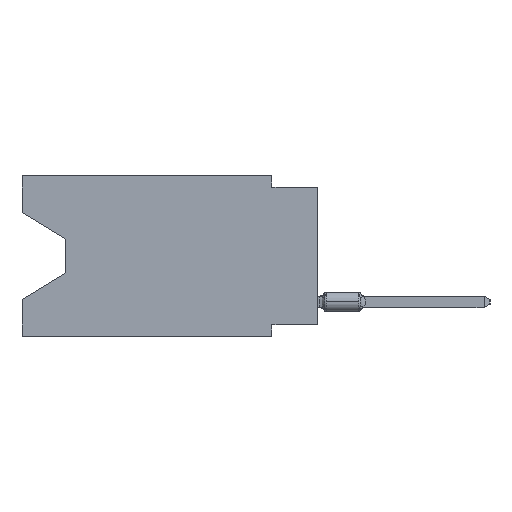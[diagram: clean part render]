
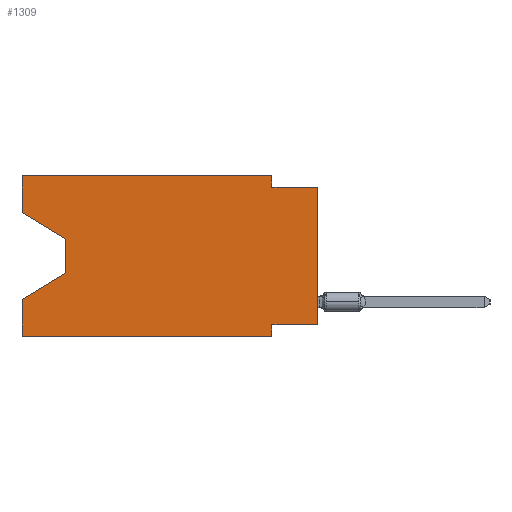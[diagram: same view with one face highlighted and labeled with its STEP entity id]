
A CAD part, left-side view. The second image highlights one B-rep face of the part: STEP entity #1309.
In plain terms, the highlighted planar face has unit normal (-1, 0, 0).
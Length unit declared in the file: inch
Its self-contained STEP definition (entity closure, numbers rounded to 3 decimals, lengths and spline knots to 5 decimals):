
#181 = ORIENTED_EDGE ( 'NONE', *, *, #13323, .T. ) ;
#307 = VECTOR ( 'NONE', #14241, 39.37008 ) ;
#564 = CARTESIAN_POINT ( 'NONE',  ( 0., 0., -0.325 ) ) ;
#871 = DIRECTION ( 'NONE',  ( 0., 0., -1. ) ) ;
#1221 = ORIENTED_EDGE ( 'NONE', *, *, #9438, .F. ) ;
#1309 = ADVANCED_FACE ( 'NONE', ( #15555 ), #1521, .F. ) ;
#1516 = EDGE_LOOP ( 'NONE', ( #21024, #16676, #6185, #19109, #11508, #5400, #8200, #181, #15451, #1221, #11687, #3195 ) ) ;
#1521 = PLANE ( 'NONE',  #21108 ) ;
#1613 = VECTOR ( 'NONE', #12825, 39.37008 ) ;
#1845 = LINE ( 'NONE', #20956, #19260 ) ;
#2079 = DIRECTION ( 'NONE',  ( 0., 0., -1. ) ) ;
#2118 = VECTOR ( 'NONE', #14619, 39.37008 ) ;
#2159 = LINE ( 'NONE', #7213, #307 ) ;
#2301 = CARTESIAN_POINT ( 'NONE',  ( 0., 0., -0.325 ) ) ;
#2612 = VERTEX_POINT ( 'NONE', #21653 ) ;
#2760 = DIRECTION ( 'NONE',  ( 0., 0., -1. ) ) ;
#2780 = VECTOR ( 'NONE', #13853, 39.37008 ) ;
#2837 = EDGE_CURVE ( 'NONE', #18678, #20106, #11973, .T. ) ;
#3013 = CARTESIAN_POINT ( 'NONE',  ( 0., 0.55, -0.212 ) ) ;
#3195 = ORIENTED_EDGE ( 'NONE', *, *, #2837, .F. ) ;
#3665 = CARTESIAN_POINT ( 'NONE',  ( 0., 0.1, -0.35 ) ) ;
#3809 = VECTOR ( 'NONE', #22788, 39.37008 ) ;
#3866 = VERTEX_POINT ( 'NONE', #10988 ) ;
#4415 = CARTESIAN_POINT ( 'NONE',  ( 0., 0.645, -0.26975 ) ) ;
#4478 = VECTOR ( 'NONE', #4640, 39.37008 ) ;
#4485 = DIRECTION ( 'NONE',  ( 0., -1., 0. ) ) ;
#4640 = DIRECTION ( 'NONE',  ( 0., 0., -1. ) ) ;
#5290 = DIRECTION ( 'NONE',  ( 0., -0.855, -0.519 ) ) ;
#5293 = EDGE_CURVE ( 'NONE', #9256, #19907, #11342, .T. ) ;
#5400 = ORIENTED_EDGE ( 'NONE', *, *, #7651, .F. ) ;
#5637 = LINE ( 'NONE', #15893, #22373 ) ;
#6131 = VECTOR ( 'NONE', #13792, 39.37008 ) ;
#6185 = ORIENTED_EDGE ( 'NONE', *, *, #18871, .T. ) ;
#6203 = VERTEX_POINT ( 'NONE', #7719 ) ;
#6368 = VERTEX_POINT ( 'NONE', #3665 ) ;
#7213 = CARTESIAN_POINT ( 'NONE',  ( 0., 0.55, -0.212 ) ) ;
#7296 = CARTESIAN_POINT ( 'NONE',  ( 0., 0.1, 0. ) ) ;
#7651 = EDGE_CURVE ( 'NONE', #10401, #6368, #5637, .T. ) ;
#7719 = CARTESIAN_POINT ( 'NONE',  ( 0., 0.1, -0.025 ) ) ;
#7851 = LINE ( 'NONE', #16500, #1613 ) ;
#7866 = EDGE_CURVE ( 'NONE', #20106, #14023, #15283, .T. ) ;
#8200 = ORIENTED_EDGE ( 'NONE', *, *, #20249, .F. ) ;
#8267 = LINE ( 'NONE', #20369, #8464 ) ;
#8464 = VECTOR ( 'NONE', #4485, 39.37008 ) ;
#8554 = CARTESIAN_POINT ( 'NONE',  ( 0., 0., 0. ) ) ;
#9256 = VERTEX_POINT ( 'NONE', #20714 ) ;
#9433 = VERTEX_POINT ( 'NONE', #564 ) ;
#9438 = EDGE_CURVE ( 'NONE', #14023, #6203, #16571, .T. ) ;
#10234 = CARTESIAN_POINT ( 'NONE',  ( 0., 0.645, 0. ) ) ;
#10401 = VERTEX_POINT ( 'NONE', #17309 ) ;
#10988 = CARTESIAN_POINT ( 'NONE',  ( 0., 0., -0.025 ) ) ;
#11066 = LINE ( 'NONE', #2301, #2118 ) ;
#11263 = EDGE_CURVE ( 'NONE', #2612, #6368, #8267, .T. ) ;
#11342 = LINE ( 'NONE', #22258, #4478 ) ;
#11508 = ORIENTED_EDGE ( 'NONE', *, *, #11263, .T. ) ;
#11687 = ORIENTED_EDGE ( 'NONE', *, *, #7866, .F. ) ;
#11973 = LINE ( 'NONE', #20702, #3809 ) ;
#12028 = LINE ( 'NONE', #8554, #2780 ) ;
#12166 = EDGE_CURVE ( 'NONE', #18678, #9256, #1845, .T. ) ;
#12452 = CARTESIAN_POINT ( 'NONE',  ( 0., 0.645, 0. ) ) ;
#12825 = DIRECTION ( 'NONE',  ( 0., -1., 0. ) ) ;
#13207 = VECTOR ( 'NONE', #13673, 39.37008 ) ;
#13323 = EDGE_CURVE ( 'NONE', #9433, #3866, #12028, .T. ) ;
#13673 = DIRECTION ( 'NONE',  ( 0., -1., 0. ) ) ;
#13792 = DIRECTION ( 'NONE',  ( 0., 0., 1. ) ) ;
#13853 = DIRECTION ( 'NONE',  ( 0., 0., 1. ) ) ;
#14023 = VERTEX_POINT ( 'NONE', #7296 ) ;
#14241 = DIRECTION ( 'NONE',  ( 0., 0.855, -0.519 ) ) ;
#14619 = DIRECTION ( 'NONE',  ( 0., 1., 0. ) ) ;
#15283 = LINE ( 'NONE', #22314, #13207 ) ;
#15451 = ORIENTED_EDGE ( 'NONE', *, *, #22483, .F. ) ;
#15555 = FACE_OUTER_BOUND ( 'NONE', #1516, .T. ) ;
#15893 = CARTESIAN_POINT ( 'NONE',  ( 0., 0.1, -0.35 ) ) ;
#16339 = CARTESIAN_POINT ( 'NONE',  ( 0., 0.1, 0. ) ) ;
#16500 = CARTESIAN_POINT ( 'NONE',  ( 0., 0., -0.025 ) ) ;
#16571 = LINE ( 'NONE', #16339, #17259 ) ;
#16676 = ORIENTED_EDGE ( 'NONE', *, *, #5293, .T. ) ;
#17259 = VECTOR ( 'NONE', #2760, 39.37008 ) ;
#17298 = CARTESIAN_POINT ( 'NONE',  ( 0., 0.645, 0. ) ) ;
#17309 = CARTESIAN_POINT ( 'NONE',  ( 0., 0.1, -0.325 ) ) ;
#17419 = EDGE_CURVE ( 'NONE', #2612, #20983, #20809, .T. ) ;
#18678 = VERTEX_POINT ( 'NONE', #20812 ) ;
#18792 = DIRECTION ( 'NONE',  ( 1., 0., 0. ) ) ;
#18871 = EDGE_CURVE ( 'NONE', #19907, #20983, #2159, .T. ) ;
#19109 = ORIENTED_EDGE ( 'NONE', *, *, #17419, .F. ) ;
#19260 = VECTOR ( 'NONE', #5290, 39.37008 ) ;
#19907 = VERTEX_POINT ( 'NONE', #3013 ) ;
#20106 = VERTEX_POINT ( 'NONE', #12452 ) ;
#20249 = EDGE_CURVE ( 'NONE', #9433, #10401, #11066, .T. ) ;
#20369 = CARTESIAN_POINT ( 'NONE',  ( 0., 0.645, -0.35 ) ) ;
#20702 = CARTESIAN_POINT ( 'NONE',  ( 0., 0.645, 0. ) ) ;
#20714 = CARTESIAN_POINT ( 'NONE',  ( 0., 0.55, -0.138 ) ) ;
#20809 = LINE ( 'NONE', #10234, #6131 ) ;
#20812 = CARTESIAN_POINT ( 'NONE',  ( 0., 0.645, -0.08025 ) ) ;
#20956 = CARTESIAN_POINT ( 'NONE',  ( 0., 0.645, -0.08025 ) ) ;
#20983 = VERTEX_POINT ( 'NONE', #4415 ) ;
#21024 = ORIENTED_EDGE ( 'NONE', *, *, #12166, .T. ) ;
#21108 = AXIS2_PLACEMENT_3D ( 'NONE', #17298, #18792, #871 ) ;
#21653 = CARTESIAN_POINT ( 'NONE',  ( 0., 0.645, -0.35 ) ) ;
#22258 = CARTESIAN_POINT ( 'NONE',  ( 0., 0.55, -0.138 ) ) ;
#22314 = CARTESIAN_POINT ( 'NONE',  ( 0., 0.645, 0. ) ) ;
#22373 = VECTOR ( 'NONE', #2079, 39.37008 ) ;
#22483 = EDGE_CURVE ( 'NONE', #6203, #3866, #7851, .T. ) ;
#22788 = DIRECTION ( 'NONE',  ( 0., 0., 1. ) ) ;
